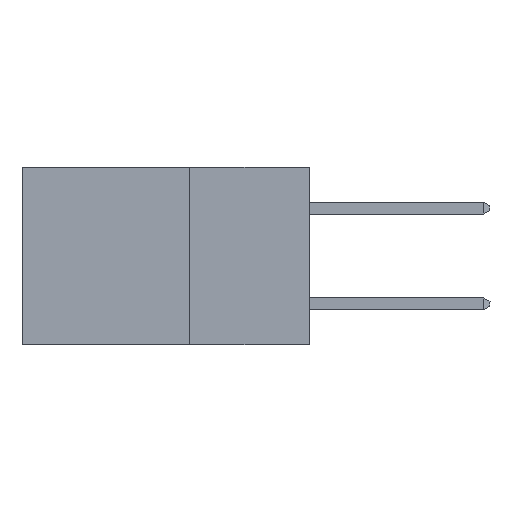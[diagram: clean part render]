
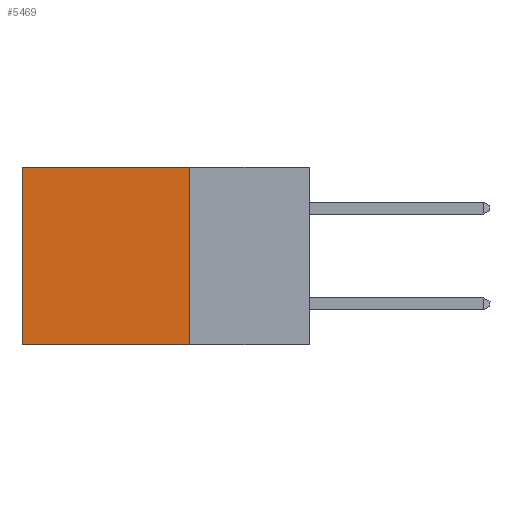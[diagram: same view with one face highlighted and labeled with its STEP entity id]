
A CAD part, left-side view. The second image highlights one B-rep face of the part: STEP entity #5469.
In plain terms, the highlighted planar face has unit normal (-1, 0, 0).
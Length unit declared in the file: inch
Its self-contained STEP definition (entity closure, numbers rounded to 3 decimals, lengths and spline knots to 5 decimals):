
#397 = CARTESIAN_POINT ( 'NONE',  ( 0.2875, 0.25, 0. ) ) ;
#447 = EDGE_CURVE ( 'NONE', #1701, #9649, #8128, .T. ) ;
#584 = LINE ( 'NONE', #9220, #8978 ) ;
#719 = DIRECTION ( 'NONE',  ( 0., 0., -1. ) ) ;
#795 = DIRECTION ( 'NONE',  ( 0., 0., -1. ) ) ;
#861 = ORIENTED_EDGE ( 'NONE', *, *, #447, .T. ) ;
#1049 = DIRECTION ( 'NONE',  ( 0., 1., 0. ) ) ;
#1451 = DIRECTION ( 'NONE',  ( 0., 1., 0. ) ) ;
#1674 = LINE ( 'NONE', #2937, #6067 ) ;
#1701 = VERTEX_POINT ( 'NONE', #2850 ) ;
#2850 = CARTESIAN_POINT ( 'NONE',  ( 0.2875, 0.6, 0. ) ) ;
#2900 = VECTOR ( 'NONE', #7396, 39.37008 ) ;
#2937 = CARTESIAN_POINT ( 'NONE',  ( 0.2875, 0.25, -0.37 ) ) ;
#2968 = VECTOR ( 'NONE', #719, 39.37008 ) ;
#3420 = PLANE ( 'NONE',  #7665 ) ;
#4058 = VERTEX_POINT ( 'NONE', #4628 ) ;
#4140 = LINE ( 'NONE', #397, #2968 ) ;
#4628 = CARTESIAN_POINT ( 'NONE',  ( 0.2875, 0.25, -0.37 ) ) ;
#4781 = ORIENTED_EDGE ( 'NONE', *, *, #11135, .F. ) ;
#5469 = ADVANCED_FACE ( 'NONE', ( #8603 ), #3420, .F. ) ;
#5599 = ORIENTED_EDGE ( 'NONE', *, *, #10070, .T. ) ;
#5850 = CARTESIAN_POINT ( 'NONE',  ( 0.2875, 0.6, -0.37 ) ) ;
#6067 = VECTOR ( 'NONE', #1049, 39.37008 ) ;
#6726 = CARTESIAN_POINT ( 'NONE',  ( 0.2875, 0.25, 0. ) ) ;
#7381 = VERTEX_POINT ( 'NONE', #10516 ) ;
#7396 = DIRECTION ( 'NONE',  ( 0., 0., -1. ) ) ;
#7498 = CARTESIAN_POINT ( 'NONE',  ( 0.2875, 0.6, 0. ) ) ;
#7665 = AXIS2_PLACEMENT_3D ( 'NONE', #6726, #10385, #795 ) ;
#7898 = EDGE_LOOP ( 'NONE', ( #861, #4781, #10960, #5599 ) ) ;
#8128 = LINE ( 'NONE', #7498, #2900 ) ;
#8603 = FACE_OUTER_BOUND ( 'NONE', #7898, .T. ) ;
#8978 = VECTOR ( 'NONE', #1451, 39.37008 ) ;
#9220 = CARTESIAN_POINT ( 'NONE',  ( 0.2875, 0.25, 0. ) ) ;
#9649 = VERTEX_POINT ( 'NONE', #5850 ) ;
#10070 = EDGE_CURVE ( 'NONE', #7381, #1701, #584, .T. ) ;
#10385 = DIRECTION ( 'NONE',  ( 1., 0., 0. ) ) ;
#10460 = EDGE_CURVE ( 'NONE', #7381, #4058, #4140, .T. ) ;
#10516 = CARTESIAN_POINT ( 'NONE',  ( 0.2875, 0.25, 0. ) ) ;
#10960 = ORIENTED_EDGE ( 'NONE', *, *, #10460, .F. ) ;
#11135 = EDGE_CURVE ( 'NONE', #4058, #9649, #1674, .T. ) ;
